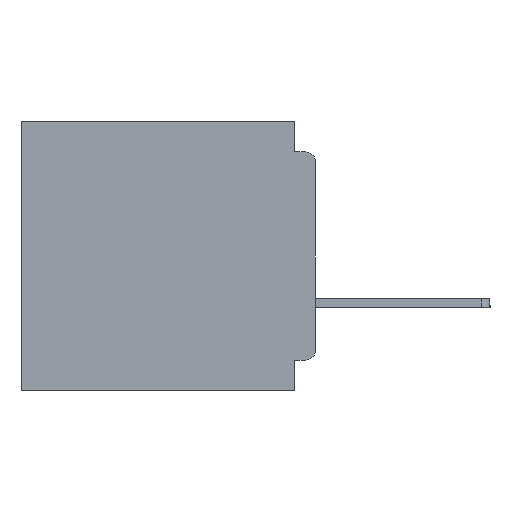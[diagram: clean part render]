
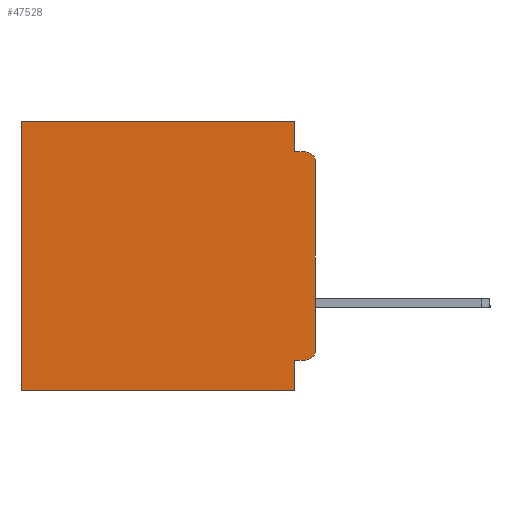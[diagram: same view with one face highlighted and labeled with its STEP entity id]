
A CAD part, left-side view. The second image highlights one B-rep face of the part: STEP entity #47528.
In plain terms, the highlighted planar face has unit normal (-1, 0, 0).
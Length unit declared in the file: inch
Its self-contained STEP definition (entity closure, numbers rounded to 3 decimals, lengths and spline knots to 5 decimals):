
#1798 = VECTOR ( 'NONE', #14292, 39.37008 ) ;
#3449 = VERTEX_POINT ( 'NONE', #15281 ) ;
#3931 = DIRECTION ( 'NONE',  ( 0., 0., -1. ) ) ;
#4096 = VERTEX_POINT ( 'NONE', #15067 ) ;
#4265 = VERTEX_POINT ( 'NONE', #17030 ) ;
#4453 = CARTESIAN_POINT ( 'NONE',  ( 0.3, 0., -0.4 ) ) ;
#4762 = VERTEX_POINT ( 'NONE', #30858 ) ;
#5129 = EDGE_LOOP ( 'NONE', ( #22100, #34222, #15746, #20381, #14024, #36035, #7560, #27323, #20992, #31976 ) ) ;
#5177 = CARTESIAN_POINT ( 'NONE',  ( 0.3, 0.031, -0.4 ) ) ;
#5518 = VERTEX_POINT ( 'NONE', #15343 ) ;
#5771 = CARTESIAN_POINT ( 'NONE',  ( 0.3, 0., -0.355 ) ) ;
#6505 = EDGE_CURVE ( 'NONE', #5518, #4265, #31443, .T. ) ;
#6734 = CARTESIAN_POINT ( 'NONE',  ( 0.3, 0., -0.045 ) ) ;
#7404 = CARTESIAN_POINT ( 'NONE',  ( 0.3, 0.015, -0.06 ) ) ;
#7560 = ORIENTED_EDGE ( 'NONE', *, *, #37139, .F. ) ;
#7843 = AXIS2_PLACEMENT_3D ( 'NONE', #4453, #30446, #8188 ) ;
#8188 = DIRECTION ( 'NONE',  ( 0., 0., -1. ) ) ;
#8490 = CARTESIAN_POINT ( 'NONE',  ( 0.3, 0., -0.34 ) ) ;
#10725 = EDGE_CURVE ( 'NONE', #4096, #37584, #18197, .T. ) ;
#10829 = CARTESIAN_POINT ( 'NONE',  ( 0.3, 0.031, 0. ) ) ;
#11004 = LINE ( 'NONE', #43970, #20911 ) ;
#11170 = DIRECTION ( 'NONE',  ( 0., 0., -1. ) ) ;
#11678 = DIRECTION ( 'NONE',  ( -1., 0., 0. ) ) ;
#12343 = VERTEX_POINT ( 'NONE', #29407 ) ;
#13921 = VECTOR ( 'NONE', #32898, 39.37008 ) ;
#14024 = ORIENTED_EDGE ( 'NONE', *, *, #32292, .T. ) ;
#14292 = DIRECTION ( 'NONE',  ( 0., -1., 0. ) ) ;
#14619 = DIRECTION ( 'NONE',  ( 0., 0., -1. ) ) ;
#15067 = CARTESIAN_POINT ( 'NONE',  ( 0.3, 0.031, -0.355 ) ) ;
#15281 = CARTESIAN_POINT ( 'NONE',  ( 0.3, 0.031, 0. ) ) ;
#15343 = CARTESIAN_POINT ( 'NONE',  ( 0.3, 0.031, -0.045 ) ) ;
#15622 = EDGE_CURVE ( 'NONE', #12343, #34063, #30110, .T. ) ;
#15746 = ORIENTED_EDGE ( 'NONE', *, *, #6505, .F. ) ;
#16115 = DIRECTION ( 'NONE',  ( 0., 1., 0. ) ) ;
#16626 = AXIS2_PLACEMENT_3D ( 'NONE', #7404, #33334, #11170 ) ;
#17030 = CARTESIAN_POINT ( 'NONE',  ( 0.3, 0.015, -0.045 ) ) ;
#17714 = CIRCLE ( 'NONE', #16626, 0.015 ) ;
#18197 = LINE ( 'NONE', #5177, #46535 ) ;
#19093 = VECTOR ( 'NONE', #3931, 39.37008 ) ;
#20381 = ORIENTED_EDGE ( 'NONE', *, *, #25641, .F. ) ;
#20685 = LINE ( 'NONE', #30813, #29364 ) ;
#20911 = VECTOR ( 'NONE', #32772, 39.37008 ) ;
#20992 = ORIENTED_EDGE ( 'NONE', *, *, #33228, .F. ) ;
#22100 = ORIENTED_EDGE ( 'NONE', *, *, #15622, .F. ) ;
#22465 = CARTESIAN_POINT ( 'NONE',  ( 0.3, 0., -0.4 ) ) ;
#22540 = LINE ( 'NONE', #10829, #23692 ) ;
#22996 = PLANE ( 'NONE',  #7843 ) ;
#23587 = EDGE_CURVE ( 'NONE', #32356, #34063, #25637, .T. ) ;
#23692 = VECTOR ( 'NONE', #14619, 39.37008 ) ;
#25120 = EDGE_CURVE ( 'NONE', #4762, #27599, #43435, .T. ) ;
#25637 = CIRCLE ( 'NONE', #33154, 0.015 ) ;
#25641 = EDGE_CURVE ( 'NONE', #3449, #5518, #22540, .T. ) ;
#27323 = ORIENTED_EDGE ( 'NONE', *, *, #10725, .F. ) ;
#27437 = DIRECTION ( 'NONE',  ( 0., 0., -1. ) ) ;
#27599 = VERTEX_POINT ( 'NONE', #34291 ) ;
#29364 = VECTOR ( 'NONE', #16115, 39.37008 ) ;
#29407 = CARTESIAN_POINT ( 'NONE',  ( 0.3, 0., -0.06 ) ) ;
#30110 = LINE ( 'NONE', #22465, #19093 ) ;
#30446 = DIRECTION ( 'NONE',  ( 1., 0., 0. ) ) ;
#30813 = CARTESIAN_POINT ( 'NONE',  ( 0.3, 0., -0.4 ) ) ;
#30858 = CARTESIAN_POINT ( 'NONE',  ( 0.3, 0.437, 0. ) ) ;
#31443 = LINE ( 'NONE', #6734, #1798 ) ;
#31976 = ORIENTED_EDGE ( 'NONE', *, *, #23587, .T. ) ;
#32292 = EDGE_CURVE ( 'NONE', #3449, #4762, #11004, .T. ) ;
#32356 = VERTEX_POINT ( 'NONE', #40697 ) ;
#32772 = DIRECTION ( 'NONE',  ( 0., 1., 0. ) ) ;
#32898 = DIRECTION ( 'NONE',  ( 0., 0., -1. ) ) ;
#33154 = AXIS2_PLACEMENT_3D ( 'NONE', #33837, #11678, #37601 ) ;
#33228 = EDGE_CURVE ( 'NONE', #32356, #4096, #47627, .T. ) ;
#33334 = DIRECTION ( 'NONE',  ( -1., 0., 0. ) ) ;
#33837 = CARTESIAN_POINT ( 'NONE',  ( 0.3, 0.015, -0.34 ) ) ;
#33996 = FACE_OUTER_BOUND ( 'NONE', #5129, .T. ) ;
#34063 = VERTEX_POINT ( 'NONE', #8490 ) ;
#34222 = ORIENTED_EDGE ( 'NONE', *, *, #41592, .T. ) ;
#34291 = CARTESIAN_POINT ( 'NONE',  ( 0.3, 0.437, -0.4 ) ) ;
#36035 = ORIENTED_EDGE ( 'NONE', *, *, #25120, .T. ) ;
#36649 = VECTOR ( 'NONE', #46467, 39.37008 ) ;
#37139 = EDGE_CURVE ( 'NONE', #37584, #27599, #20685, .T. ) ;
#37584 = VERTEX_POINT ( 'NONE', #48084 ) ;
#37601 = DIRECTION ( 'NONE',  ( 0., 0., -1. ) ) ;
#40190 = CARTESIAN_POINT ( 'NONE',  ( 0.3, 0.437, -0.4 ) ) ;
#40697 = CARTESIAN_POINT ( 'NONE',  ( 0.3, 0.015, -0.355 ) ) ;
#41592 = EDGE_CURVE ( 'NONE', #12343, #4265, #17714, .T. ) ;
#43435 = LINE ( 'NONE', #40190, #13921 ) ;
#43970 = CARTESIAN_POINT ( 'NONE',  ( 0.3, 0., 0. ) ) ;
#46467 = DIRECTION ( 'NONE',  ( 0., 1., 0. ) ) ;
#46535 = VECTOR ( 'NONE', #27437, 39.37008 ) ;
#47528 = ADVANCED_FACE ( 'NONE', ( #33996 ), #22996, .F. ) ;
#47627 = LINE ( 'NONE', #5771, #36649 ) ;
#48084 = CARTESIAN_POINT ( 'NONE',  ( 0.3, 0.031, -0.4 ) ) ;
